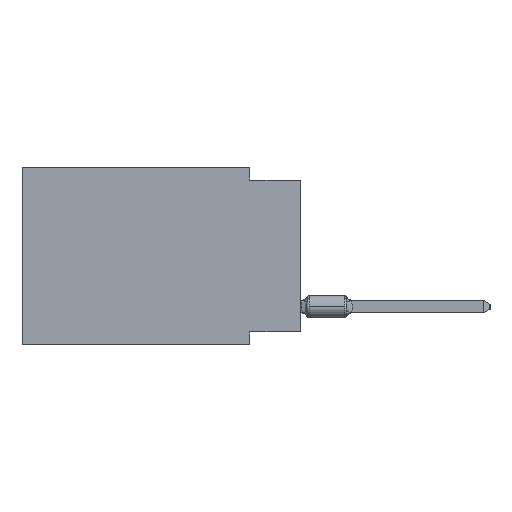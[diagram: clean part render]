
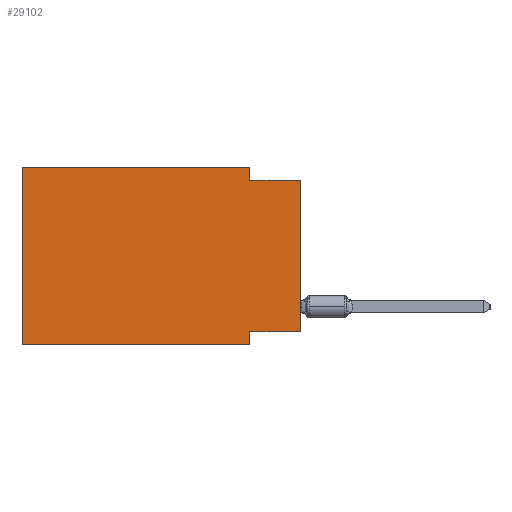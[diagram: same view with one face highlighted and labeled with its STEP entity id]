
A CAD part, left-side view. The second image highlights one B-rep face of the part: STEP entity #29102.
In plain terms, the highlighted planar face has unit normal (-1, 0, 0).
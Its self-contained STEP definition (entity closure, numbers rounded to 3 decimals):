
#1176 = DIRECTION ( 'NONE',  ( 0., 0., -1. ) ) ;
#1310 = EDGE_CURVE ( 'NONE', #30826, #26045, #34057, .T. ) ;
#1848 = DIRECTION ( 'NONE',  ( 0., 0., -1. ) ) ;
#2537 = ORIENTED_EDGE ( 'NONE', *, *, #30625, .F. ) ;
#2717 = CARTESIAN_POINT ( 'NONE',  ( 0., 13.97, 0. ) ) ;
#2828 = ORIENTED_EDGE ( 'NONE', *, *, #47071, .F. ) ;
#2855 = DIRECTION ( 'NONE',  ( 0., -1., 0. ) ) ;
#3107 = VERTEX_POINT ( 'NONE', #13153 ) ;
#3572 = LINE ( 'NONE', #36696, #11694 ) ;
#4700 = CARTESIAN_POINT ( 'NONE',  ( 0., 13.97, 0. ) ) ;
#4921 = ORIENTED_EDGE ( 'NONE', *, *, #26077, .F. ) ;
#7480 = DIRECTION ( 'NONE',  ( 0., 0., 1. ) ) ;
#8801 = DIRECTION ( 'NONE',  ( 1., 0., 0. ) ) ;
#8933 = VERTEX_POINT ( 'NONE', #2717 ) ;
#8978 = LINE ( 'NONE', #4700, #26758 ) ;
#9079 = VECTOR ( 'NONE', #7480, 1000. ) ;
#10108 = DIRECTION ( 'NONE',  ( 0., -1., 0. ) ) ;
#11267 = CARTESIAN_POINT ( 'NONE',  ( 0., 13.97, 0. ) ) ;
#11690 = VECTOR ( 'NONE', #40599, 1000. ) ;
#11694 = VECTOR ( 'NONE', #2855, 1000. ) ;
#11980 = VERTEX_POINT ( 'NONE', #13947 ) ;
#12835 = ORIENTED_EDGE ( 'NONE', *, *, #31679, .F. ) ;
#13153 = CARTESIAN_POINT ( 'NONE',  ( 0., 0., -0.635 ) ) ;
#13947 = CARTESIAN_POINT ( 'NONE',  ( 0., 2.54, -0.635 ) ) ;
#15777 = DIRECTION ( 'NONE',  ( 0., 0., -1. ) ) ;
#15953 = DIRECTION ( 'NONE',  ( 0., -1., 0. ) ) ;
#16040 = CARTESIAN_POINT ( 'NONE',  ( 0., 2.54, -8.89 ) ) ;
#16688 = ORIENTED_EDGE ( 'NONE', *, *, #40702, .T. ) ;
#18428 = CARTESIAN_POINT ( 'NONE',  ( 0., 2.54, -8.89 ) ) ;
#18437 = ORIENTED_EDGE ( 'NONE', *, *, #27664, .F. ) ;
#18661 = LINE ( 'NONE', #44848, #20130 ) ;
#20130 = VECTOR ( 'NONE', #15777, 1000. ) ;
#21779 = CARTESIAN_POINT ( 'NONE',  ( 0., 0., -8.255 ) ) ;
#24386 = FACE_OUTER_BOUND ( 'NONE', #28493, .T. ) ;
#25180 = VERTEX_POINT ( 'NONE', #46963 ) ;
#25998 = EDGE_CURVE ( 'NONE', #37492, #26045, #3572, .T. ) ;
#26045 = VERTEX_POINT ( 'NONE', #18428 ) ;
#26077 = EDGE_CURVE ( 'NONE', #25180, #11980, #18661, .T. ) ;
#26758 = VECTOR ( 'NONE', #15953, 1000. ) ;
#27514 = CARTESIAN_POINT ( 'NONE',  ( 0., 13.97, 0. ) ) ;
#27664 = EDGE_CURVE ( 'NONE', #37492, #8933, #32902, .T. ) ;
#28493 = EDGE_LOOP ( 'NONE', ( #16688, #2537, #4921, #12835, #18437, #34309, #46178, #2828 ) ) ;
#29102 = ADVANCED_FACE ( 'NONE', ( #24386 ), #41722, .F. ) ;
#30625 = EDGE_CURVE ( 'NONE', #11980, #3107, #39425, .T. ) ;
#30826 = VERTEX_POINT ( 'NONE', #34081 ) ;
#31381 = VERTEX_POINT ( 'NONE', #42653 ) ;
#31679 = EDGE_CURVE ( 'NONE', #8933, #25180, #8978, .T. ) ;
#32164 = VECTOR ( 'NONE', #10108, 1000. ) ;
#32902 = LINE ( 'NONE', #11267, #11690 ) ;
#33295 = LINE ( 'NONE', #21779, #37274 ) ;
#34057 = LINE ( 'NONE', #16040, #39009 ) ;
#34081 = CARTESIAN_POINT ( 'NONE',  ( 0., 2.54, -8.255 ) ) ;
#34309 = ORIENTED_EDGE ( 'NONE', *, *, #25998, .T. ) ;
#36402 = AXIS2_PLACEMENT_3D ( 'NONE', #27514, #8801, #1848 ) ;
#36696 = CARTESIAN_POINT ( 'NONE',  ( 0., 13.97, -8.89 ) ) ;
#37238 = CARTESIAN_POINT ( 'NONE',  ( 0., 0., 0. ) ) ;
#37274 = VECTOR ( 'NONE', #39584, 1000. ) ;
#37492 = VERTEX_POINT ( 'NONE', #44999 ) ;
#39009 = VECTOR ( 'NONE', #1176, 1000. ) ;
#39425 = LINE ( 'NONE', #43016, #32164 ) ;
#39584 = DIRECTION ( 'NONE',  ( 0., 1., 0. ) ) ;
#40393 = LINE ( 'NONE', #37238, #9079 ) ;
#40599 = DIRECTION ( 'NONE',  ( 0., 0., 1. ) ) ;
#40702 = EDGE_CURVE ( 'NONE', #31381, #3107, #40393, .T. ) ;
#41722 = PLANE ( 'NONE',  #36402 ) ;
#42653 = CARTESIAN_POINT ( 'NONE',  ( 0., 0., -8.255 ) ) ;
#43016 = CARTESIAN_POINT ( 'NONE',  ( 0., 0., -0.635 ) ) ;
#44848 = CARTESIAN_POINT ( 'NONE',  ( 0., 2.54, 0. ) ) ;
#44999 = CARTESIAN_POINT ( 'NONE',  ( 0., 13.97, -8.89 ) ) ;
#46178 = ORIENTED_EDGE ( 'NONE', *, *, #1310, .F. ) ;
#46963 = CARTESIAN_POINT ( 'NONE',  ( 0., 2.54, 0. ) ) ;
#47071 = EDGE_CURVE ( 'NONE', #31381, #30826, #33295, .T. ) ;
